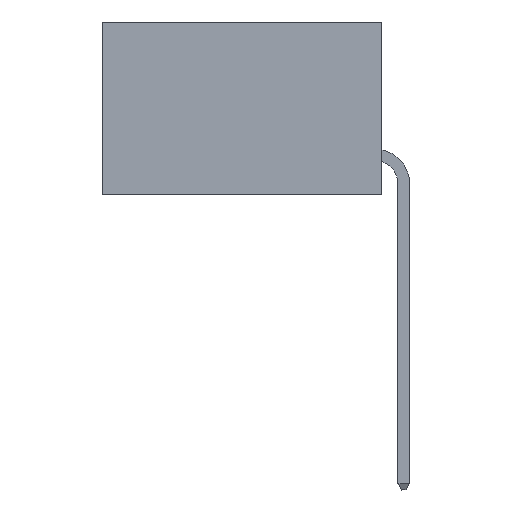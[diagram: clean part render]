
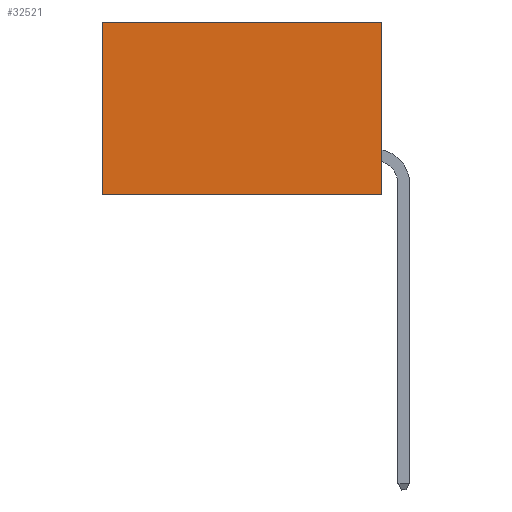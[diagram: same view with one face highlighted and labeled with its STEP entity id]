
A CAD part, left-side view. The second image highlights one B-rep face of the part: STEP entity #32521.
In plain terms, the highlighted planar face has unit normal (-1, 0, 0).
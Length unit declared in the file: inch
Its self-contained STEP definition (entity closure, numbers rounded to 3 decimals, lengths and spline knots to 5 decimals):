
#913 = VECTOR ( 'NONE', #17060, 39.37008 ) ;
#1232 = DIRECTION ( 'NONE',  ( 0., 0., -1. ) ) ;
#5624 = EDGE_CURVE ( 'NONE', #26365, #26773, #32366, .T. ) ;
#6123 = ORIENTED_EDGE ( 'NONE', *, *, #43513, .F. ) ;
#8386 = FACE_OUTER_BOUND ( 'NONE', #24121, .T. ) ;
#14015 = CARTESIAN_POINT ( 'NONE',  ( 0.2875, 0.6, -0.37 ) ) ;
#15025 = CARTESIAN_POINT ( 'NONE',  ( 0.2875, 0., -0.37 ) ) ;
#15118 = LINE ( 'NONE', #23525, #27929 ) ;
#16219 = VERTEX_POINT ( 'NONE', #14015 ) ;
#17060 = DIRECTION ( 'NONE',  ( 0., 0., -1. ) ) ;
#22954 = VERTEX_POINT ( 'NONE', #15025 ) ;
#23104 = EDGE_CURVE ( 'NONE', #26773, #16219, #15118, .T. ) ;
#23525 = CARTESIAN_POINT ( 'NONE',  ( 0.2875, 0.6, 0. ) ) ;
#24121 = EDGE_LOOP ( 'NONE', ( #27297, #47614, #6123, #38433 ) ) ;
#26023 = CARTESIAN_POINT ( 'NONE',  ( 0.2875, 0., -0.37 ) ) ;
#26365 = VERTEX_POINT ( 'NONE', #28517 ) ;
#26773 = VERTEX_POINT ( 'NONE', #45830 ) ;
#27271 = EDGE_CURVE ( 'NONE', #22954, #16219, #44182, .T. ) ;
#27297 = ORIENTED_EDGE ( 'NONE', *, *, #23104, .T. ) ;
#27929 = VECTOR ( 'NONE', #1232, 39.37008 ) ;
#28517 = CARTESIAN_POINT ( 'NONE',  ( 0.2875, 0., 0. ) ) ;
#28627 = CARTESIAN_POINT ( 'NONE',  ( 0.2875, 0., 0. ) ) ;
#29740 = DIRECTION ( 'NONE',  ( 0., 1., 0. ) ) ;
#29770 = CARTESIAN_POINT ( 'NONE',  ( 0.2875, 0., 0. ) ) ;
#31212 = VECTOR ( 'NONE', #44682, 39.37008 ) ;
#31676 = PLANE ( 'NONE',  #43469 ) ;
#32366 = LINE ( 'NONE', #29770, #31212 ) ;
#32521 = ADVANCED_FACE ( 'NONE', ( #8386 ), #31676, .F. ) ;
#33148 = VECTOR ( 'NONE', #29740, 39.37008 ) ;
#35394 = DIRECTION ( 'NONE',  ( 1., 0., 0. ) ) ;
#38433 = ORIENTED_EDGE ( 'NONE', *, *, #5624, .T. ) ;
#39148 = DIRECTION ( 'NONE',  ( 0., 0., -1. ) ) ;
#43469 = AXIS2_PLACEMENT_3D ( 'NONE', #46773, #35394, #39148 ) ;
#43513 = EDGE_CURVE ( 'NONE', #26365, #22954, #46806, .T. ) ;
#44182 = LINE ( 'NONE', #26023, #33148 ) ;
#44682 = DIRECTION ( 'NONE',  ( 0., 1., 0. ) ) ;
#45830 = CARTESIAN_POINT ( 'NONE',  ( 0.2875, 0.6, 0. ) ) ;
#46773 = CARTESIAN_POINT ( 'NONE',  ( 0.2875, 0., 0. ) ) ;
#46806 = LINE ( 'NONE', #28627, #913 ) ;
#47614 = ORIENTED_EDGE ( 'NONE', *, *, #27271, .F. ) ;
